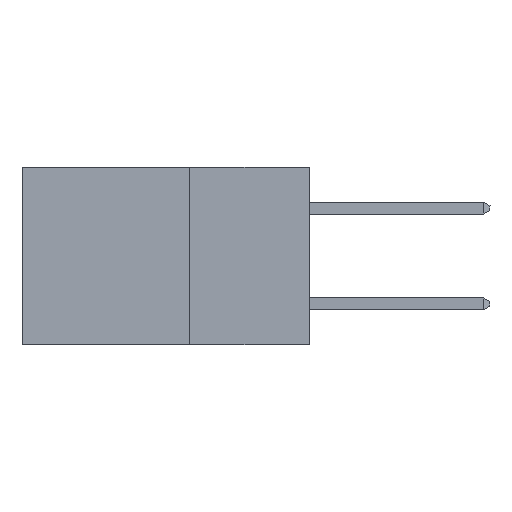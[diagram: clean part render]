
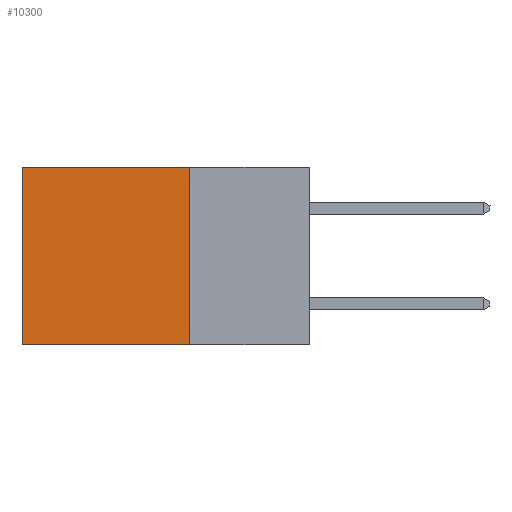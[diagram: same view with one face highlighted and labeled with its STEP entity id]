
A CAD part, left-side view. The second image highlights one B-rep face of the part: STEP entity #10300.
In plain terms, the highlighted planar face has unit normal (-1, 0, 0).
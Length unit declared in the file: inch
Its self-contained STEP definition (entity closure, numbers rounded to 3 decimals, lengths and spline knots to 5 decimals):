
#106 = EDGE_CURVE ( 'NONE', #4742, #6658, #5016, .T. ) ;
#175 = VECTOR ( 'NONE', #10099, 39.37008 ) ;
#961 = EDGE_CURVE ( 'NONE', #13048, #3845, #8207, .T. ) ;
#1795 = CARTESIAN_POINT ( 'NONE',  ( 0.2875, 0.25, 0. ) ) ;
#1915 = ORIENTED_EDGE ( 'NONE', *, *, #10134, .T. ) ;
#2498 = CARTESIAN_POINT ( 'NONE',  ( 0.2875, 0.6, 0. ) ) ;
#2911 = VECTOR ( 'NONE', #6119, 39.37008 ) ;
#3184 = DIRECTION ( 'NONE',  ( 1., 0., 0. ) ) ;
#3392 = LINE ( 'NONE', #9001, #175 ) ;
#3414 = FACE_OUTER_BOUND ( 'NONE', #7559, .T. ) ;
#3845 = VERTEX_POINT ( 'NONE', #13789 ) ;
#4418 = CARTESIAN_POINT ( 'NONE',  ( 0.2875, 0.25, -0.37 ) ) ;
#4483 = ORIENTED_EDGE ( 'NONE', *, *, #11935, .F. ) ;
#4742 = VERTEX_POINT ( 'NONE', #6910 ) ;
#5016 = LINE ( 'NONE', #1795, #13993 ) ;
#5324 = VECTOR ( 'NONE', #12246, 39.37008 ) ;
#6119 = DIRECTION ( 'NONE',  ( 0., 1., 0. ) ) ;
#6504 = ORIENTED_EDGE ( 'NONE', *, *, #106, .F. ) ;
#6658 = VERTEX_POINT ( 'NONE', #4418 ) ;
#6910 = CARTESIAN_POINT ( 'NONE',  ( 0.2875, 0.25, 0. ) ) ;
#7196 = DIRECTION ( 'NONE',  ( 0., 0., -1. ) ) ;
#7499 = CARTESIAN_POINT ( 'NONE',  ( 0.2875, 0.25, 0. ) ) ;
#7559 = EDGE_LOOP ( 'NONE', ( #12565, #4483, #6504, #1915 ) ) ;
#8207 = LINE ( 'NONE', #2498, #5324 ) ;
#8569 = AXIS2_PLACEMENT_3D ( 'NONE', #7499, #3184, #10764 ) ;
#9001 = CARTESIAN_POINT ( 'NONE',  ( 0.2875, 0.25, -0.37 ) ) ;
#9673 = PLANE ( 'NONE',  #8569 ) ;
#10099 = DIRECTION ( 'NONE',  ( 0., 1., 0. ) ) ;
#10134 = EDGE_CURVE ( 'NONE', #4742, #13048, #13745, .T. ) ;
#10300 = ADVANCED_FACE ( 'NONE', ( #3414 ), #9673, .F. ) ;
#10764 = DIRECTION ( 'NONE',  ( 0., 0., -1. ) ) ;
#11935 = EDGE_CURVE ( 'NONE', #6658, #3845, #3392, .T. ) ;
#11958 = CARTESIAN_POINT ( 'NONE',  ( 0.2875, 0.6, 0. ) ) ;
#12246 = DIRECTION ( 'NONE',  ( 0., 0., -1. ) ) ;
#12565 = ORIENTED_EDGE ( 'NONE', *, *, #961, .T. ) ;
#12607 = CARTESIAN_POINT ( 'NONE',  ( 0.2875, 0.25, 0. ) ) ;
#13048 = VERTEX_POINT ( 'NONE', #11958 ) ;
#13745 = LINE ( 'NONE', #12607, #2911 ) ;
#13789 = CARTESIAN_POINT ( 'NONE',  ( 0.2875, 0.6, -0.37 ) ) ;
#13993 = VECTOR ( 'NONE', #7196, 39.37008 ) ;
